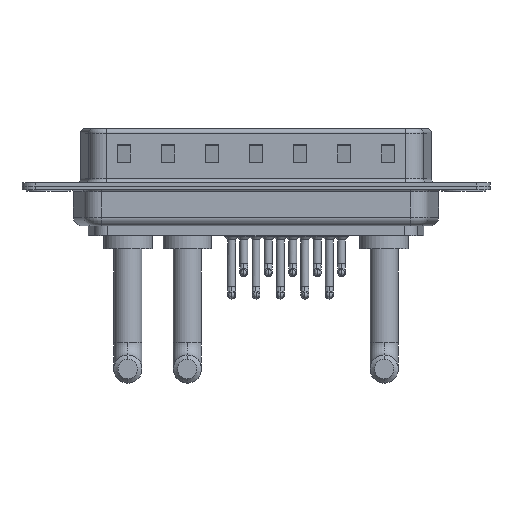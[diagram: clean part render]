
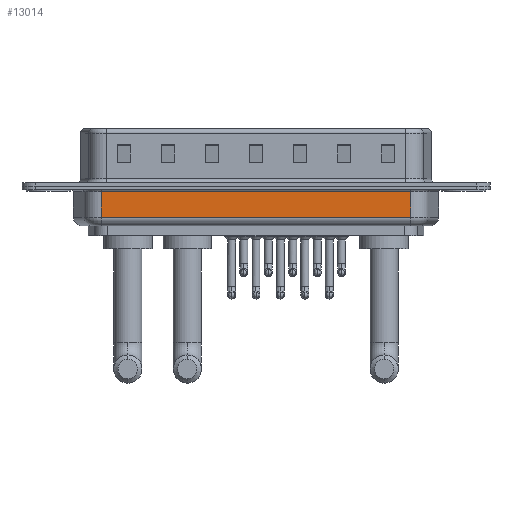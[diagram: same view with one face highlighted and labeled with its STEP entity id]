
A CAD part, front view. The second image highlights one B-rep face of the part: STEP entity #13014.
In plain terms, the highlighted planar face has unit normal (0, -1, 0).
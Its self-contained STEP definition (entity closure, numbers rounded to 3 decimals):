
#540 = CARTESIAN_POINT ( 'NONE',  ( 41.044, -5.35, -0.65 ) ) ;
#644 = EDGE_CURVE ( 'NONE', #1659, #2193, #15850, .T. ) ;
#767 = DIRECTION ( 'NONE',  ( 0., 0., 1. ) ) ;
#1094 = CARTESIAN_POINT ( 'NONE',  ( 41.044, -5.35, -4.5 ) ) ;
#1642 = CARTESIAN_POINT ( 'NONE',  ( 6.006, -5.35, -4.5 ) ) ;
#1659 = VERTEX_POINT ( 'NONE', #12703 ) ;
#1892 = AXIS2_PLACEMENT_3D ( 'NONE', #1642, #14658, #4975 ) ;
#2193 = VERTEX_POINT ( 'NONE', #8465 ) ;
#2407 = LINE ( 'NONE', #5844, #3338 ) ;
#2498 = CARTESIAN_POINT ( 'NONE',  ( 6.006, -5.35, -0.65 ) ) ;
#3243 = ORIENTED_EDGE ( 'NONE', *, *, #14965, .T. ) ;
#3338 = VECTOR ( 'NONE', #14413, 1000. ) ;
#3391 = VECTOR ( 'NONE', #12276, 1000. ) ;
#3557 = VECTOR ( 'NONE', #767, 1000. ) ;
#3868 = ORIENTED_EDGE ( 'NONE', *, *, #5195, .T. ) ;
#4657 = CARTESIAN_POINT ( 'NONE',  ( 41.044, -5.35, -3.5 ) ) ;
#4755 = FACE_OUTER_BOUND ( 'NONE', #14717, .T. ) ;
#4975 = DIRECTION ( 'NONE',  ( 0., 0., 1. ) ) ;
#5195 = EDGE_CURVE ( 'NONE', #1659, #18047, #2407, .T. ) ;
#5742 = CARTESIAN_POINT ( 'NONE',  ( 6.006, -5.35, -4.5 ) ) ;
#5844 = CARTESIAN_POINT ( 'NONE',  ( 6.006, -5.35, -3.5 ) ) ;
#5924 = LINE ( 'NONE', #2498, #3391 ) ;
#8211 = VECTOR ( 'NONE', #19392, 1000. ) ;
#8465 = CARTESIAN_POINT ( 'NONE',  ( 6.006, -5.35, -0.65 ) ) ;
#8469 = EDGE_CURVE ( 'NONE', #18047, #21511, #19505, .T. ) ;
#12276 = DIRECTION ( 'NONE',  ( -1., 0., 0. ) ) ;
#12703 = CARTESIAN_POINT ( 'NONE',  ( 6.006, -5.35, -3.5 ) ) ;
#13014 = ADVANCED_FACE ( 'NONE', ( #4755 ), #21706, .F. ) ;
#14413 = DIRECTION ( 'NONE',  ( 1., 0., 0. ) ) ;
#14658 = DIRECTION ( 'NONE',  ( 0., 1., 0. ) ) ;
#14717 = EDGE_LOOP ( 'NONE', ( #20366, #3868, #21424, #3243 ) ) ;
#14965 = EDGE_CURVE ( 'NONE', #21511, #2193, #5924, .T. ) ;
#15850 = LINE ( 'NONE', #5742, #3557 ) ;
#18047 = VERTEX_POINT ( 'NONE', #4657 ) ;
#19392 = DIRECTION ( 'NONE',  ( 0., 0., 1. ) ) ;
#19505 = LINE ( 'NONE', #1094, #8211 ) ;
#20366 = ORIENTED_EDGE ( 'NONE', *, *, #644, .F. ) ;
#21424 = ORIENTED_EDGE ( 'NONE', *, *, #8469, .T. ) ;
#21511 = VERTEX_POINT ( 'NONE', #540 ) ;
#21706 = PLANE ( 'NONE',  #1892 ) ;
